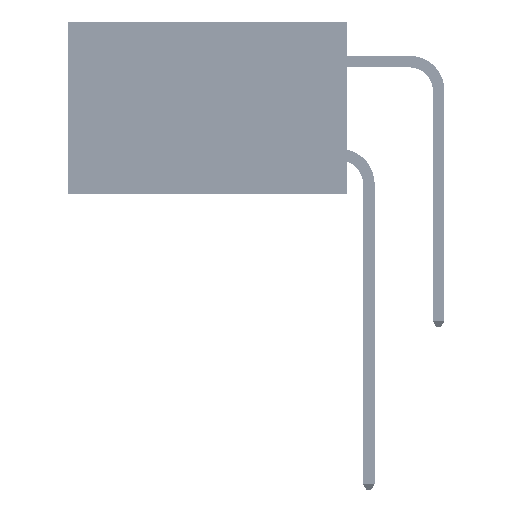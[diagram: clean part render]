
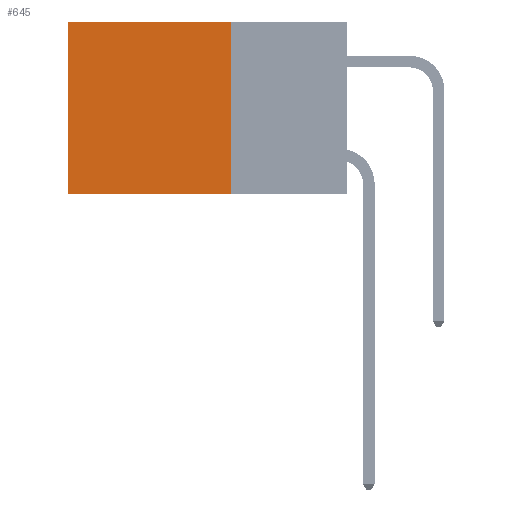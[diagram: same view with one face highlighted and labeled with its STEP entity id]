
A CAD part, left-side view. The second image highlights one B-rep face of the part: STEP entity #645.
In plain terms, the highlighted planar face has unit normal (-1, 0, 0).
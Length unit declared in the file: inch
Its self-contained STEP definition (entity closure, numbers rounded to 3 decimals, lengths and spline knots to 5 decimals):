
#342 = CARTESIAN_POINT ( 'NONE',  ( 0.2875, 0.6, -0.37 ) ) ;
#645 = ADVANCED_FACE ( 'NONE', ( #32460 ), #41202, .F. ) ;
#4911 = CARTESIAN_POINT ( 'NONE',  ( 0.2875, 0.25, -0.37 ) ) ;
#6043 = EDGE_LOOP ( 'NONE', ( #6131, #13147, #30960, #23924 ) ) ;
#6131 = ORIENTED_EDGE ( 'NONE', *, *, #24184, .T. ) ;
#8884 = CARTESIAN_POINT ( 'NONE',  ( 0.2875, 0.6, 0. ) ) ;
#12361 = VECTOR ( 'NONE', #46116, 39.37008 ) ;
#13147 = ORIENTED_EDGE ( 'NONE', *, *, #31331, .F. ) ;
#14710 = VERTEX_POINT ( 'NONE', #15338 ) ;
#15338 = CARTESIAN_POINT ( 'NONE',  ( 0.2875, 0.6, 0. ) ) ;
#18992 = CARTESIAN_POINT ( 'NONE',  ( 0.2875, 0.25, 0. ) ) ;
#22203 = CARTESIAN_POINT ( 'NONE',  ( 0.2875, 0.25, -0.37 ) ) ;
#22780 = AXIS2_PLACEMENT_3D ( 'NONE', #30289, #29631, #26274 ) ;
#23924 = ORIENTED_EDGE ( 'NONE', *, *, #27419, .T. ) ;
#24184 = EDGE_CURVE ( 'NONE', #14710, #24571, #37813, .T. ) ;
#24571 = VERTEX_POINT ( 'NONE', #342 ) ;
#26274 = DIRECTION ( 'NONE',  ( 0., 0., -1. ) ) ;
#27419 = EDGE_CURVE ( 'NONE', #47568, #14710, #42289, .T. ) ;
#27797 = VERTEX_POINT ( 'NONE', #22203 ) ;
#29631 = DIRECTION ( 'NONE',  ( 1., 0., 0. ) ) ;
#30289 = CARTESIAN_POINT ( 'NONE',  ( 0.2875, 0.25, 0. ) ) ;
#30960 = ORIENTED_EDGE ( 'NONE', *, *, #39831, .F. ) ;
#31224 = VECTOR ( 'NONE', #47582, 39.37008 ) ;
#31331 = EDGE_CURVE ( 'NONE', #27797, #24571, #46120, .T. ) ;
#31977 = DIRECTION ( 'NONE',  ( 0., 1., 0. ) ) ;
#32460 = FACE_OUTER_BOUND ( 'NONE', #6043, .T. ) ;
#32790 = LINE ( 'NONE', #18992, #12361 ) ;
#35773 = DIRECTION ( 'NONE',  ( 0., 1., 0. ) ) ;
#37813 = LINE ( 'NONE', #8884, #31224 ) ;
#39831 = EDGE_CURVE ( 'NONE', #47568, #27797, #32790, .T. ) ;
#39848 = CARTESIAN_POINT ( 'NONE',  ( 0.2875, 0.25, 0. ) ) ;
#39973 = CARTESIAN_POINT ( 'NONE',  ( 0.2875, 0.25, 0. ) ) ;
#40156 = VECTOR ( 'NONE', #35773, 39.37008 ) ;
#41202 = PLANE ( 'NONE',  #22780 ) ;
#42289 = LINE ( 'NONE', #39848, #43465 ) ;
#43465 = VECTOR ( 'NONE', #31977, 39.37008 ) ;
#46116 = DIRECTION ( 'NONE',  ( 0., 0., -1. ) ) ;
#46120 = LINE ( 'NONE', #4911, #40156 ) ;
#47568 = VERTEX_POINT ( 'NONE', #39973 ) ;
#47582 = DIRECTION ( 'NONE',  ( 0., 0., -1. ) ) ;
